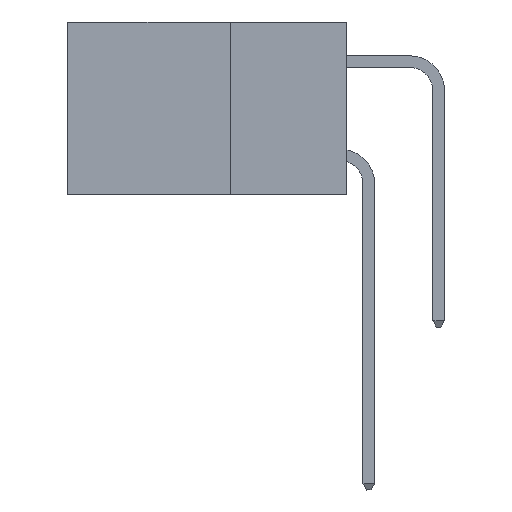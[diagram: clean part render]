
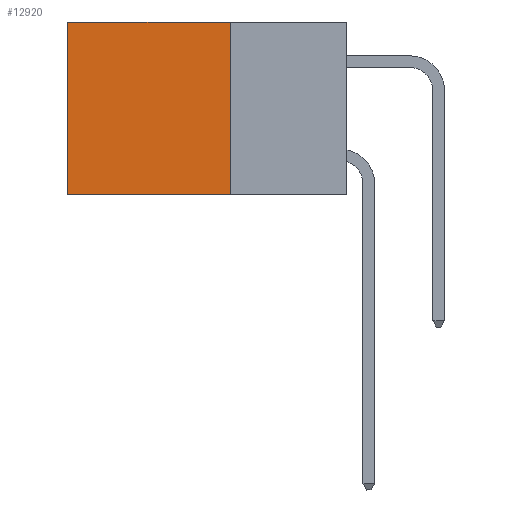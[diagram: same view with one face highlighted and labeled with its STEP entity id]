
A CAD part, left-side view. The second image highlights one B-rep face of the part: STEP entity #12920.
In plain terms, the highlighted planar face has unit normal (-1, 0, 0).
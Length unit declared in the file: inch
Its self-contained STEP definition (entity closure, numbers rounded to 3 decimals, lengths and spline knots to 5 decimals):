
#1251 = FACE_OUTER_BOUND ( 'NONE', #12688, .T. ) ;
#1926 = VERTEX_POINT ( 'NONE', #3812 ) ;
#2028 = CARTESIAN_POINT ( 'NONE',  ( 0.2875, 0.25, 0. ) ) ;
#2595 = ORIENTED_EDGE ( 'NONE', *, *, #4593, .T. ) ;
#2771 = EDGE_CURVE ( 'NONE', #1926, #16756, #4638, .T. ) ;
#3356 = CARTESIAN_POINT ( 'NONE',  ( 0.2875, 0.25, -0.37 ) ) ;
#3389 = CARTESIAN_POINT ( 'NONE',  ( 0.2875, 0.6, -0.37 ) ) ;
#3812 = CARTESIAN_POINT ( 'NONE',  ( 0.2875, 0.25, 0. ) ) ;
#4452 = CARTESIAN_POINT ( 'NONE',  ( 0.2875, 0.25, 0. ) ) ;
#4484 = LINE ( 'NONE', #11687, #15282 ) ;
#4593 = EDGE_CURVE ( 'NONE', #1926, #12251, #13435, .T. ) ;
#4638 = LINE ( 'NONE', #19734, #11920 ) ;
#4840 = EDGE_CURVE ( 'NONE', #16756, #5379, #17854, .T. ) ;
#5379 = VERTEX_POINT ( 'NONE', #3389 ) ;
#5380 = VECTOR ( 'NONE', #11761, 39.37008 ) ;
#6141 = ORIENTED_EDGE ( 'NONE', *, *, #2771, .F. ) ;
#11687 = CARTESIAN_POINT ( 'NONE',  ( 0.2875, 0.6, 0. ) ) ;
#11761 = DIRECTION ( 'NONE',  ( 0., 1., 0. ) ) ;
#11920 = VECTOR ( 'NONE', #13324, 39.37008 ) ;
#12251 = VERTEX_POINT ( 'NONE', #20232 ) ;
#12688 = EDGE_LOOP ( 'NONE', ( #12868, #15470, #6141, #2595 ) ) ;
#12868 = ORIENTED_EDGE ( 'NONE', *, *, #14634, .T. ) ;
#12920 = ADVANCED_FACE ( 'NONE', ( #1251 ), #18844, .F. ) ;
#13324 = DIRECTION ( 'NONE',  ( 0., 0., -1. ) ) ;
#13435 = LINE ( 'NONE', #2028, #5380 ) ;
#14393 = CARTESIAN_POINT ( 'NONE',  ( 0.2875, 0.25, -0.37 ) ) ;
#14581 = DIRECTION ( 'NONE',  ( 0., 1., 0. ) ) ;
#14634 = EDGE_CURVE ( 'NONE', #12251, #5379, #4484, .T. ) ;
#15182 = DIRECTION ( 'NONE',  ( 0., 0., -1. ) ) ;
#15282 = VECTOR ( 'NONE', #15182, 39.37008 ) ;
#15346 = VECTOR ( 'NONE', #14581, 39.37008 ) ;
#15470 = ORIENTED_EDGE ( 'NONE', *, *, #4840, .F. ) ;
#15695 = DIRECTION ( 'NONE',  ( 1., 0., 0. ) ) ;
#16756 = VERTEX_POINT ( 'NONE', #14393 ) ;
#17401 = AXIS2_PLACEMENT_3D ( 'NONE', #4452, #15695, #17455 ) ;
#17455 = DIRECTION ( 'NONE',  ( 0., 0., -1. ) ) ;
#17854 = LINE ( 'NONE', #3356, #15346 ) ;
#18844 = PLANE ( 'NONE',  #17401 ) ;
#19734 = CARTESIAN_POINT ( 'NONE',  ( 0.2875, 0.25, 0. ) ) ;
#20232 = CARTESIAN_POINT ( 'NONE',  ( 0.2875, 0.6, 0. ) ) ;
